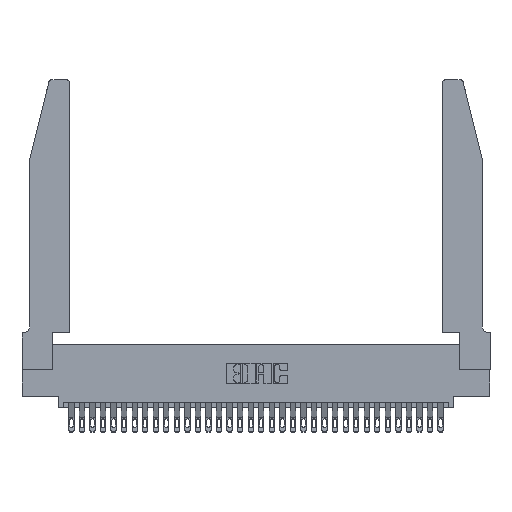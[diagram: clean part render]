
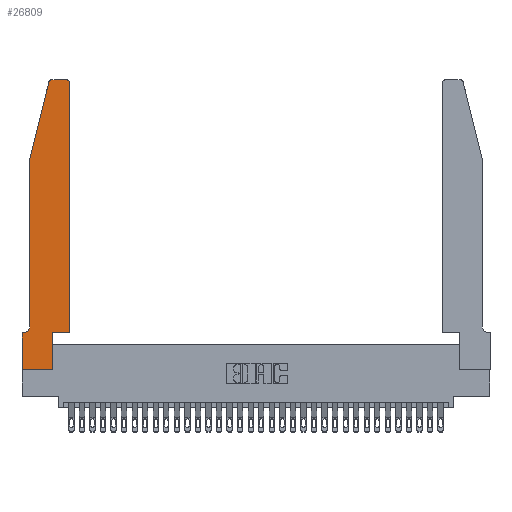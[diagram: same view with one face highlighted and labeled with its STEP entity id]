
A CAD part, top view. The second image highlights one B-rep face of the part: STEP entity #26809.
In plain terms, the highlighted planar face has unit normal (0, 0, 1).
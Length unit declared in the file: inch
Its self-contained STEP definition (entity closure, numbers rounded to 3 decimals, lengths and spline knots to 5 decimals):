
#20 = LINE ( 'NONE', #12045, #13331 ) ;
#985 = CIRCLE ( 'NONE', #21767, 0.03 ) ;
#1064 = ORIENTED_EDGE ( 'NONE', *, *, #11411, .T. ) ;
#1576 = VERTEX_POINT ( 'NONE', #5475 ) ;
#1814 = CARTESIAN_POINT ( 'NONE',  ( 0.4505, 0.35, 0.37 ) ) ;
#2033 = CARTESIAN_POINT ( 'NONE',  ( 0.2865, 0.35, 0.37 ) ) ;
#2228 = AXIS2_PLACEMENT_3D ( 'NONE', #10722, #31889, #2710 ) ;
#2710 = DIRECTION ( 'NONE',  ( 1., 0., 0. ) ) ;
#2910 = AXIS2_PLACEMENT_3D ( 'NONE', #9812, #28355, #12454 ) ;
#2914 = CARTESIAN_POINT ( 'NONE',  ( 0.4505, 0.35, 0.37 ) ) ;
#3173 = LINE ( 'NONE', #7333, #7760 ) ;
#3817 = DIRECTION ( 'NONE',  ( -1., 0., 0. ) ) ;
#3897 = VERTEX_POINT ( 'NONE', #23628 ) ;
#4780 = LINE ( 'NONE', #6926, #18042 ) ;
#5459 = DIRECTION ( 'NONE',  ( 0., -1., 0. ) ) ;
#5475 = CARTESIAN_POINT ( 'NONE',  ( 0.0755, 0.42, 0.37 ) ) ;
#5893 = DIRECTION ( 'NONE',  ( -1., 0., 0. ) ) ;
#6187 = CARTESIAN_POINT ( 'NONE',  ( 0.284, 2.72, 0.37 ) ) ;
#6760 = VECTOR ( 'NONE', #5459, 39.37008 ) ;
#6926 = CARTESIAN_POINT ( 'NONE',  ( 0.0755, 2., 0.37 ) ) ;
#6957 = ORIENTED_EDGE ( 'NONE', *, *, #26573, .T. ) ;
#7333 = CARTESIAN_POINT ( 'NONE',  ( 0., 0., 0.37 ) ) ;
#7557 = DIRECTION ( 'NONE',  ( 1., 0., 0. ) ) ;
#7627 = EDGE_CURVE ( 'NONE', #12670, #14609, #19947, .T. ) ;
#7676 = VERTEX_POINT ( 'NONE', #2914 ) ;
#7760 = VECTOR ( 'NONE', #23426, 39.37008 ) ;
#7979 = EDGE_CURVE ( 'NONE', #28040, #33892, #20, .T. ) ;
#8131 = VERTEX_POINT ( 'NONE', #30885 ) ;
#8496 = CIRCLE ( 'NONE', #2910, 0.03 ) ;
#8997 = DIRECTION ( 'NONE',  ( 1., 0., 0. ) ) ;
#9278 = CARTESIAN_POINT ( 'NONE',  ( 0.2865, 0.35, 0.37 ) ) ;
#9760 = DIRECTION ( 'NONE',  ( 0., 1., 0. ) ) ;
#9812 = CARTESIAN_POINT ( 'NONE',  ( 0.4205, 2.72, 0.37 ) ) ;
#10083 = ORIENTED_EDGE ( 'NONE', *, *, #7627, .T. ) ;
#10584 = ORIENTED_EDGE ( 'NONE', *, *, #25694, .T. ) ;
#10722 = CARTESIAN_POINT ( 'NONE',  ( 0., 0.35, 0.37 ) ) ;
#11022 = ORIENTED_EDGE ( 'NONE', *, *, #27788, .T. ) ;
#11188 = EDGE_CURVE ( 'NONE', #27019, #25041, #8496, .T. ) ;
#11411 = EDGE_CURVE ( 'NONE', #8131, #23450, #4780, .T. ) ;
#11449 = DIRECTION ( 'NONE',  ( 0., 0., -1. ) ) ;
#11996 = EDGE_CURVE ( 'NONE', #3897, #8131, #985, .T. ) ;
#12045 = CARTESIAN_POINT ( 'NONE',  ( 0., 0., 0.37 ) ) ;
#12367 = EDGE_CURVE ( 'NONE', #7676, #27019, #13632, .T. ) ;
#12454 = DIRECTION ( 'NONE',  ( 1., 0., 0. ) ) ;
#12585 = CARTESIAN_POINT ( 'NONE',  ( 0.4505, 2.72, 0.37 ) ) ;
#12670 = VERTEX_POINT ( 'NONE', #27261 ) ;
#12791 = DIRECTION ( 'NONE',  ( -1., 0., 0. ) ) ;
#12800 = ORIENTED_EDGE ( 'NONE', *, *, #11996, .T. ) ;
#13035 = ORIENTED_EDGE ( 'NONE', *, *, #15137, .T. ) ;
#13331 = VECTOR ( 'NONE', #30569, 39.37008 ) ;
#13632 = LINE ( 'NONE', #1814, #33104 ) ;
#13644 = LINE ( 'NONE', #15798, #20306 ) ;
#14609 = VERTEX_POINT ( 'NONE', #28107 ) ;
#15044 = DIRECTION ( 'NONE',  ( -0.239, -0.971, 0. ) ) ;
#15137 = EDGE_CURVE ( 'NONE', #1576, #12670, #26005, .T. ) ;
#15798 = CARTESIAN_POINT ( 'NONE',  ( 0.4505, 0.35, 0.37 ) ) ;
#16150 = CARTESIAN_POINT ( 'NONE',  ( 0.0755, 2., 0.37 ) ) ;
#17441 = CARTESIAN_POINT ( 'NONE',  ( 0.0755, 2., 0.37 ) ) ;
#17536 = LINE ( 'NONE', #16150, #6760 ) ;
#17613 = EDGE_CURVE ( 'NONE', #25041, #3897, #23340, .T. ) ;
#18031 = VERTEX_POINT ( 'NONE', #2033 ) ;
#18042 = VECTOR ( 'NONE', #15044, 39.37008 ) ;
#19947 = LINE ( 'NONE', #29772, #20784 ) ;
#20306 = VECTOR ( 'NONE', #7557, 39.37008 ) ;
#20519 = AXIS2_PLACEMENT_3D ( 'NONE', #22334, #11449, #3817 ) ;
#20784 = VECTOR ( 'NONE', #5893, 39.37008 ) ;
#21613 = CARTESIAN_POINT ( 'NONE',  ( 0., 0., 0.37 ) ) ;
#21767 = AXIS2_PLACEMENT_3D ( 'NONE', #6187, #32960, #8997 ) ;
#21960 = ORIENTED_EDGE ( 'NONE', *, *, #7979, .T. ) ;
#22334 = CARTESIAN_POINT ( 'NONE',  ( 0.0055, 0.42, 0.37 ) ) ;
#22699 = ORIENTED_EDGE ( 'NONE', *, *, #11188, .T. ) ;
#23050 = ORIENTED_EDGE ( 'NONE', *, *, #29559, .T. ) ;
#23201 = ORIENTED_EDGE ( 'NONE', *, *, #12367, .T. ) ;
#23229 = EDGE_LOOP ( 'NONE', ( #24040, #12800, #1064, #10584, #13035, #10083, #23050, #21960, #6957, #11022, #23201, #22699 ) ) ;
#23340 = LINE ( 'NONE', #33819, #27923 ) ;
#23426 = DIRECTION ( 'NONE',  ( 0., -1., 0. ) ) ;
#23450 = VERTEX_POINT ( 'NONE', #17441 ) ;
#23628 = CARTESIAN_POINT ( 'NONE',  ( 0.284, 2.75, 0.37 ) ) ;
#24040 = ORIENTED_EDGE ( 'NONE', *, *, #17613, .T. ) ;
#24924 = CARTESIAN_POINT ( 'NONE',  ( 0.2865, 0., 0.37 ) ) ;
#25041 = VERTEX_POINT ( 'NONE', #26290 ) ;
#25312 = DIRECTION ( 'NONE',  ( 0., 1., 0. ) ) ;
#25694 = EDGE_CURVE ( 'NONE', #23450, #1576, #17536, .T. ) ;
#26005 = CIRCLE ( 'NONE', #20519, 0.07 ) ;
#26290 = CARTESIAN_POINT ( 'NONE',  ( 0.4205, 2.75, 0.37 ) ) ;
#26573 = EDGE_CURVE ( 'NONE', #33892, #18031, #28716, .T. ) ;
#26809 = ADVANCED_FACE ( 'NONE', ( #34028 ), #32202, .T. ) ;
#27019 = VERTEX_POINT ( 'NONE', #12585 ) ;
#27261 = CARTESIAN_POINT ( 'NONE',  ( 0.0055, 0.35, 0.37 ) ) ;
#27788 = EDGE_CURVE ( 'NONE', #18031, #7676, #13644, .T. ) ;
#27923 = VECTOR ( 'NONE', #12791, 39.37008 ) ;
#28040 = VERTEX_POINT ( 'NONE', #21613 ) ;
#28107 = CARTESIAN_POINT ( 'NONE',  ( 0., 0.35, 0.37 ) ) ;
#28355 = DIRECTION ( 'NONE',  ( 0., 0., 1. ) ) ;
#28716 = LINE ( 'NONE', #9278, #31129 ) ;
#29559 = EDGE_CURVE ( 'NONE', #14609, #28040, #3173, .T. ) ;
#29772 = CARTESIAN_POINT ( 'NONE',  ( 0.0755, 0.35, 0.37 ) ) ;
#30569 = DIRECTION ( 'NONE',  ( 1., 0., 0. ) ) ;
#30885 = CARTESIAN_POINT ( 'NONE',  ( 0.25487, 2.72718, 0.37 ) ) ;
#31129 = VECTOR ( 'NONE', #9760, 39.37008 ) ;
#31889 = DIRECTION ( 'NONE',  ( 0., 0., 1. ) ) ;
#32202 = PLANE ( 'NONE',  #2228 ) ;
#32960 = DIRECTION ( 'NONE',  ( 0., 0., 1. ) ) ;
#33104 = VECTOR ( 'NONE', #25312, 39.37008 ) ;
#33819 = CARTESIAN_POINT ( 'NONE',  ( 0.2605, 2.75, 0.37 ) ) ;
#33892 = VERTEX_POINT ( 'NONE', #24924 ) ;
#34028 = FACE_OUTER_BOUND ( 'NONE', #23229, .T. ) ;
